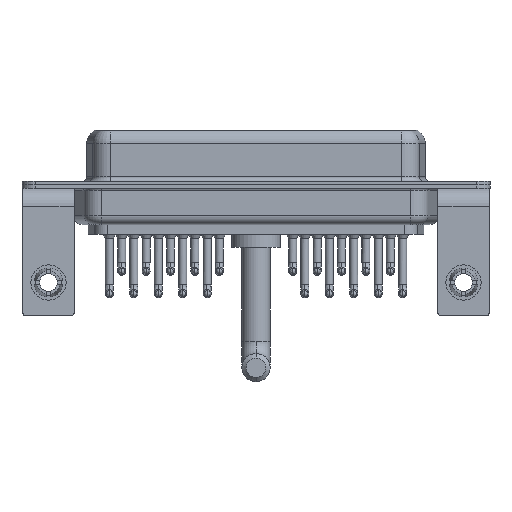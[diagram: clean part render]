
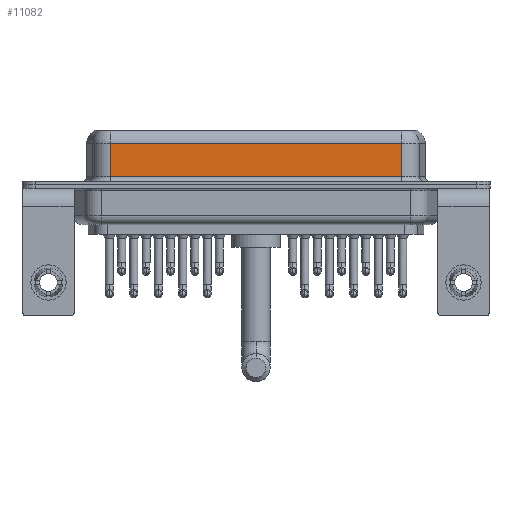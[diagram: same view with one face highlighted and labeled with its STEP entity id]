
A CAD part, front view. The second image highlights one B-rep face of the part: STEP entity #11082.
In plain terms, the highlighted planar face has unit normal (0, -1, 0).
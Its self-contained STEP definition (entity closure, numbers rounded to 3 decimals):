
#944 = CARTESIAN_POINT ( 'NONE',  ( 7.013, -3.95, 0.9 ) ) ;
#2625 = VERTEX_POINT ( 'NONE', #944 ) ;
#3632 = EDGE_CURVE ( 'NONE', #2625, #17331, #14667, .T. ) ;
#3831 = EDGE_CURVE ( 'NONE', #14159, #17331, #6832, .T. ) ;
#5145 = CARTESIAN_POINT ( 'NONE',  ( 40.037, -3.95, 0.9 ) ) ;
#6832 = LINE ( 'NONE', #20278, #19355 ) ;
#7109 = DIRECTION ( 'NONE',  ( 0., 0., -1. ) ) ;
#7218 = EDGE_CURVE ( 'NONE', #14159, #22713, #8678, .T. ) ;
#8484 = DIRECTION ( 'NONE',  ( 0., 0., -1. ) ) ;
#8678 = LINE ( 'NONE', #12966, #19112 ) ;
#8791 = DIRECTION ( 'NONE',  ( -1., 0., 0. ) ) ;
#9005 = AXIS2_PLACEMENT_3D ( 'NONE', #14224, #20440, #18422 ) ;
#9247 = CARTESIAN_POINT ( 'NONE',  ( 7.013, -3.95, 6.4 ) ) ;
#9978 = CARTESIAN_POINT ( 'NONE',  ( 40.037, -3.95, 0.9 ) ) ;
#10334 = ORIENTED_EDGE ( 'NONE', *, *, #3831, .F. ) ;
#10657 = FACE_OUTER_BOUND ( 'NONE', #13935, .T. ) ;
#11082 = ADVANCED_FACE ( 'NONE', ( #10657 ), #18041, .F. ) ;
#11486 = ORIENTED_EDGE ( 'NONE', *, *, #7218, .T. ) ;
#12966 = CARTESIAN_POINT ( 'NONE',  ( 40.037, -3.95, 4.65 ) ) ;
#13935 = EDGE_LOOP ( 'NONE', ( #10334, #11486, #24070, #16172 ) ) ;
#14159 = VERTEX_POINT ( 'NONE', #24025 ) ;
#14224 = CARTESIAN_POINT ( 'NONE',  ( 40.037, -3.95, 6.4 ) ) ;
#14667 = LINE ( 'NONE', #5145, #24235 ) ;
#16172 = ORIENTED_EDGE ( 'NONE', *, *, #3632, .T. ) ;
#17134 = EDGE_CURVE ( 'NONE', #22713, #2625, #22708, .T. ) ;
#17331 = VERTEX_POINT ( 'NONE', #9978 ) ;
#18041 = PLANE ( 'NONE',  #9005 ) ;
#18422 = DIRECTION ( 'NONE',  ( 0., 0., 1. ) ) ;
#18976 = DIRECTION ( 'NONE',  ( 1., 0., 0. ) ) ;
#19112 = VECTOR ( 'NONE', #8791, 1000. ) ;
#19355 = VECTOR ( 'NONE', #8484, 1000. ) ;
#20278 = CARTESIAN_POINT ( 'NONE',  ( 40.037, -3.95, 6.4 ) ) ;
#20440 = DIRECTION ( 'NONE',  ( 0., 1., 0. ) ) ;
#21670 = VECTOR ( 'NONE', #7109, 1000. ) ;
#22463 = CARTESIAN_POINT ( 'NONE',  ( 7.013, -3.95, 4.65 ) ) ;
#22708 = LINE ( 'NONE', #9247, #21670 ) ;
#22713 = VERTEX_POINT ( 'NONE', #22463 ) ;
#24025 = CARTESIAN_POINT ( 'NONE',  ( 40.037, -3.95, 4.65 ) ) ;
#24070 = ORIENTED_EDGE ( 'NONE', *, *, #17134, .T. ) ;
#24235 = VECTOR ( 'NONE', #18976, 1000. ) ;
